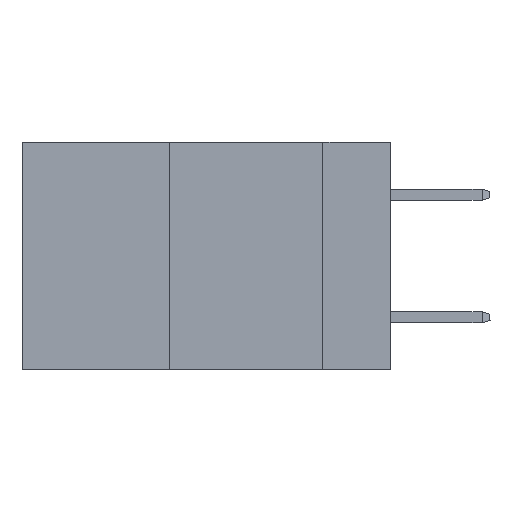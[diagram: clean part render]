
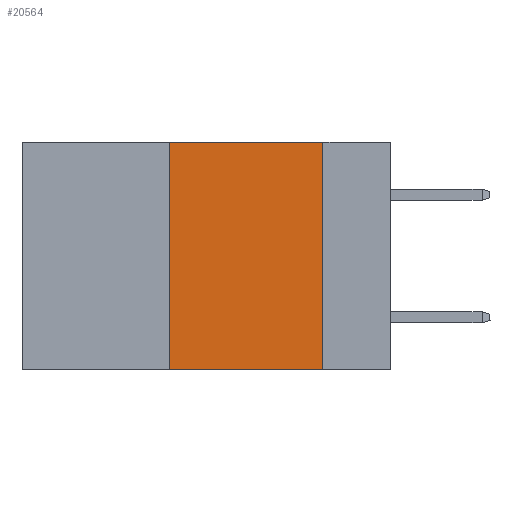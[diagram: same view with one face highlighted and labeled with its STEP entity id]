
A CAD part, left-side view. The second image highlights one B-rep face of the part: STEP entity #20564.
In plain terms, the highlighted planar face has unit normal (-1, 0, 0).
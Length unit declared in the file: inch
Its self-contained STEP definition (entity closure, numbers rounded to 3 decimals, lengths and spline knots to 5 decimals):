
#1457 = PLANE ( 'NONE',  #11211 ) ;
#1904 = VECTOR ( 'NONE', #2192, 39.37008 ) ;
#1962 = VERTEX_POINT ( 'NONE', #6478 ) ;
#2192 = DIRECTION ( 'NONE',  ( 0., -1., 0. ) ) ;
#2464 = LINE ( 'NONE', #14256, #1904 ) ;
#3023 = ORIENTED_EDGE ( 'NONE', *, *, #16380, .F. ) ;
#3250 = ORIENTED_EDGE ( 'NONE', *, *, #21032, .F. ) ;
#3290 = DIRECTION ( 'NONE',  ( 0., 0., -1. ) ) ;
#4089 = ORIENTED_EDGE ( 'NONE', *, *, #19912, .T. ) ;
#4747 = LINE ( 'NONE', #12887, #13310 ) ;
#5187 = LINE ( 'NONE', #17398, #10844 ) ;
#5981 = CARTESIAN_POINT ( 'NONE',  ( 0., 0.11, 0. ) ) ;
#6478 = CARTESIAN_POINT ( 'NONE',  ( 0., 0.36, 0. ) ) ;
#7377 = DIRECTION ( 'NONE',  ( 0., 0., -1. ) ) ;
#8089 = CARTESIAN_POINT ( 'NONE',  ( 0., 0.11, -0.37 ) ) ;
#9041 = VECTOR ( 'NONE', #17969, 39.37008 ) ;
#9578 = FACE_OUTER_BOUND ( 'NONE', #13769, .T. ) ;
#10814 = VERTEX_POINT ( 'NONE', #12252 ) ;
#10844 = VECTOR ( 'NONE', #7377, 39.37008 ) ;
#11211 = AXIS2_PLACEMENT_3D ( 'NONE', #16828, #13577, #3290 ) ;
#11365 = CARTESIAN_POINT ( 'NONE',  ( 0., 0.36, 0. ) ) ;
#11916 = VERTEX_POINT ( 'NONE', #8089 ) ;
#12252 = CARTESIAN_POINT ( 'NONE',  ( 0., 0.36, -0.37 ) ) ;
#12887 = CARTESIAN_POINT ( 'NONE',  ( 0., 0.6, -0.37 ) ) ;
#13310 = VECTOR ( 'NONE', #19516, 39.37008 ) ;
#13577 = DIRECTION ( 'NONE',  ( 1., 0., 0. ) ) ;
#13769 = EDGE_LOOP ( 'NONE', ( #19988, #3023, #3250, #4089 ) ) ;
#14256 = CARTESIAN_POINT ( 'NONE',  ( 0., 0.6, 0. ) ) ;
#16380 = EDGE_CURVE ( 'NONE', #1962, #20284, #2464, .T. ) ;
#16828 = CARTESIAN_POINT ( 'NONE',  ( 0., 0.6, 0. ) ) ;
#17398 = CARTESIAN_POINT ( 'NONE',  ( 0., 0.11, 0. ) ) ;
#17916 = LINE ( 'NONE', #11365, #9041 ) ;
#17969 = DIRECTION ( 'NONE',  ( 0., 0., 1. ) ) ;
#19516 = DIRECTION ( 'NONE',  ( 0., -1., 0. ) ) ;
#19912 = EDGE_CURVE ( 'NONE', #10814, #11916, #4747, .T. ) ;
#19988 = ORIENTED_EDGE ( 'NONE', *, *, #22102, .F. ) ;
#20284 = VERTEX_POINT ( 'NONE', #5981 ) ;
#20564 = ADVANCED_FACE ( 'NONE', ( #9578 ), #1457, .F. ) ;
#21032 = EDGE_CURVE ( 'NONE', #10814, #1962, #17916, .T. ) ;
#22102 = EDGE_CURVE ( 'NONE', #20284, #11916, #5187, .T. ) ;
